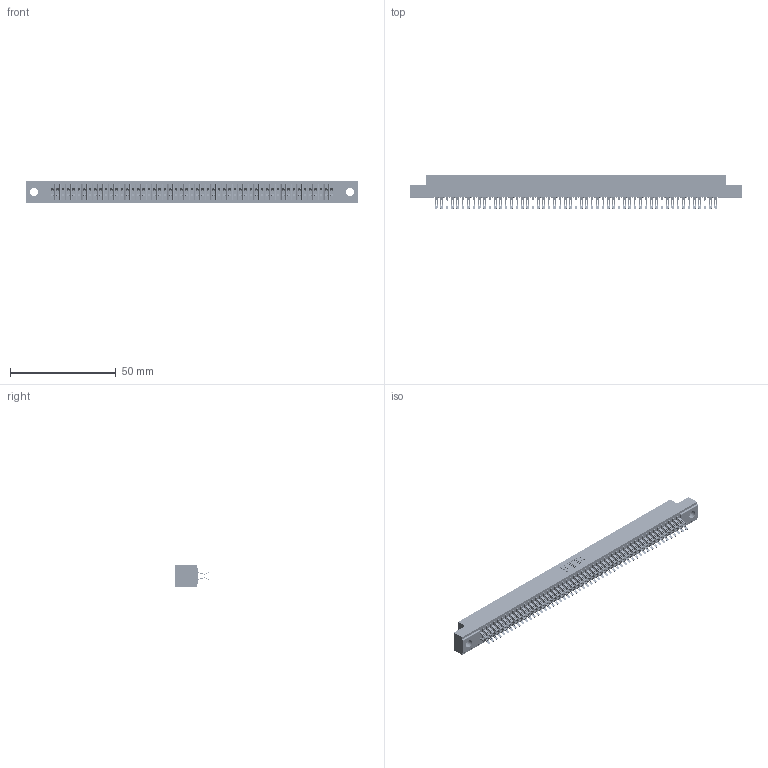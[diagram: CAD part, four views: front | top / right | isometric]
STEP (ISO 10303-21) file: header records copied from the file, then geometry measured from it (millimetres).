
FILE_DESCRIPTION (( 'STEP AP203' ), '1' );
FILE_NAME ('391-106-555-204.STEP', '2018-08-09T20:54:24', ( '' ), ( '' ), 'SwSTEP 2.0', 'SolidWorks 2016', '' );
FILE_SCHEMA (( 'CONFIG_CONTROL_DESIGN' ));
Length unit declared in the file: inch
Products named in the file (3): 341-292-001_341-292-155; 391-106-555-204; 341 Part_.156 (3.96) Dia Mounting Holes
Assembly tree (107 placements, depth 2):
  391-106-555-204
    341 Part_.156 (3.96) Dia Mounting Holes
    341-292-001_341-292-155  x106
Bounding box: 156.84 x 16.31 x 10.16 mm (x, y, z)
Volume: 11620.7 mm3; surface area: 21727 mm2
Topology: 107 solids, 107 shells, 8398 faces, 25103 edges, 16342 vertices
Faces by surface type: plane 4534, cylinder 3652, sphere 108, torus 104
Entity records: 63564 total; most frequent: CARTESIAN_POINT 10587, ORIENTED_EDGE 10510, DIRECTION 10249, EDGE_CURVE 5255, LINE 4249, VECTOR 4249, VERTEX_POINT 3322, AXIS2_PLACEMENT_3D 3000
